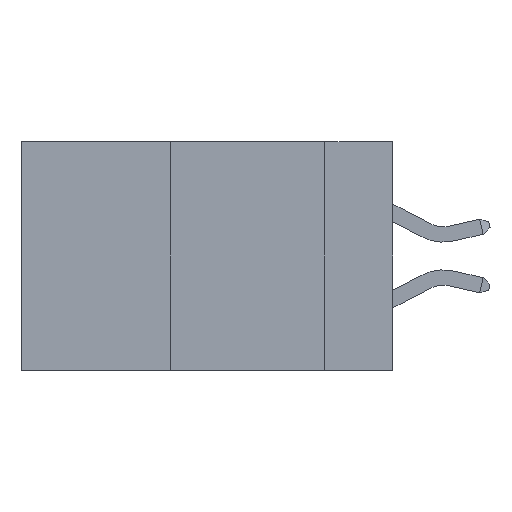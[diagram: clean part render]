
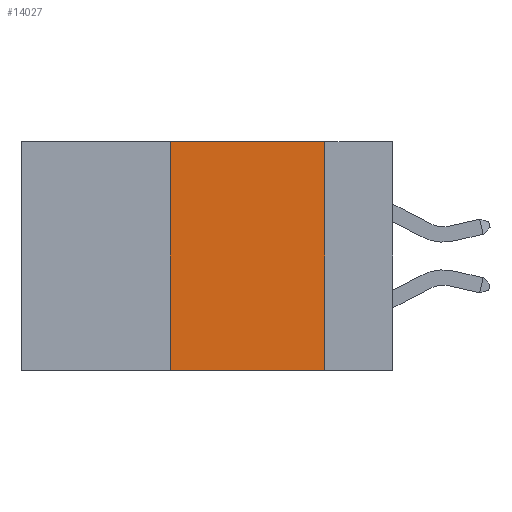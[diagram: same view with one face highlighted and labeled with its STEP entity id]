
A CAD part, left-side view. The second image highlights one B-rep face of the part: STEP entity #14027.
In plain terms, the highlighted planar face has unit normal (-1, 0, 0).
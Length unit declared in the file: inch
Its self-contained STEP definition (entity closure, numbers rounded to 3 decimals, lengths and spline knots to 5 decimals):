
#162 = EDGE_CURVE ( 'NONE', #4624, #4629, #17745, .T. ) ;
#205 = ORIENTED_EDGE ( 'NONE', *, *, #18684, .F. ) ;
#1864 = EDGE_LOOP ( 'NONE', ( #14140, #2920, #205, #11124 ) ) ;
#2596 = PLANE ( 'NONE',  #19132 ) ;
#2920 = ORIENTED_EDGE ( 'NONE', *, *, #13531, .F. ) ;
#3456 = VECTOR ( 'NONE', #4470, 39.37008 ) ;
#3870 = CARTESIAN_POINT ( 'NONE',  ( 0., 0.6, 0. ) ) ;
#4470 = DIRECTION ( 'NONE',  ( 0., 0., 1. ) ) ;
#4624 = VERTEX_POINT ( 'NONE', #11028 ) ;
#4629 = VERTEX_POINT ( 'NONE', #17651 ) ;
#4650 = CARTESIAN_POINT ( 'NONE',  ( 0., 0.6, 0. ) ) ;
#5844 = EDGE_CURVE ( 'NONE', #7137, #4629, #15167, .T. ) ;
#7137 = VERTEX_POINT ( 'NONE', #11039 ) ;
#9155 = LINE ( 'NONE', #13306, #3456 ) ;
#10459 = VERTEX_POINT ( 'NONE', #25681 ) ;
#10594 = FACE_OUTER_BOUND ( 'NONE', #1864, .T. ) ;
#11028 = CARTESIAN_POINT ( 'NONE',  ( 0., 0.11, 0. ) ) ;
#11039 = CARTESIAN_POINT ( 'NONE',  ( 0., 0.36, -0.37 ) ) ;
#11124 = ORIENTED_EDGE ( 'NONE', *, *, #5844, .T. ) ;
#11335 = VECTOR ( 'NONE', #17881, 39.37008 ) ;
#13087 = DIRECTION ( 'NONE',  ( 0., 0., -1. ) ) ;
#13306 = CARTESIAN_POINT ( 'NONE',  ( 0., 0.36, 0. ) ) ;
#13531 = EDGE_CURVE ( 'NONE', #10459, #4624, #24826, .T. ) ;
#14027 = ADVANCED_FACE ( 'NONE', ( #10594 ), #2596, .F. ) ;
#14140 = ORIENTED_EDGE ( 'NONE', *, *, #162, .F. ) ;
#15167 = LINE ( 'NONE', #18908, #21996 ) ;
#16837 = DIRECTION ( 'NONE',  ( 0., -1., 0. ) ) ;
#16838 = DIRECTION ( 'NONE',  ( 0., -1., 0. ) ) ;
#17651 = CARTESIAN_POINT ( 'NONE',  ( 0., 0.11, -0.37 ) ) ;
#17745 = LINE ( 'NONE', #26151, #11335 ) ;
#17881 = DIRECTION ( 'NONE',  ( 0., 0., -1. ) ) ;
#18684 = EDGE_CURVE ( 'NONE', #7137, #10459, #9155, .T. ) ;
#18908 = CARTESIAN_POINT ( 'NONE',  ( 0., 0.6, -0.37 ) ) ;
#19132 = AXIS2_PLACEMENT_3D ( 'NONE', #4650, #23665, #13087 ) ;
#21996 = VECTOR ( 'NONE', #16838, 39.37008 ) ;
#23665 = DIRECTION ( 'NONE',  ( 1., 0., 0. ) ) ;
#24826 = LINE ( 'NONE', #3870, #27107 ) ;
#25681 = CARTESIAN_POINT ( 'NONE',  ( 0., 0.36, 0. ) ) ;
#26151 = CARTESIAN_POINT ( 'NONE',  ( 0., 0.11, 0. ) ) ;
#27107 = VECTOR ( 'NONE', #16837, 39.37008 ) ;
